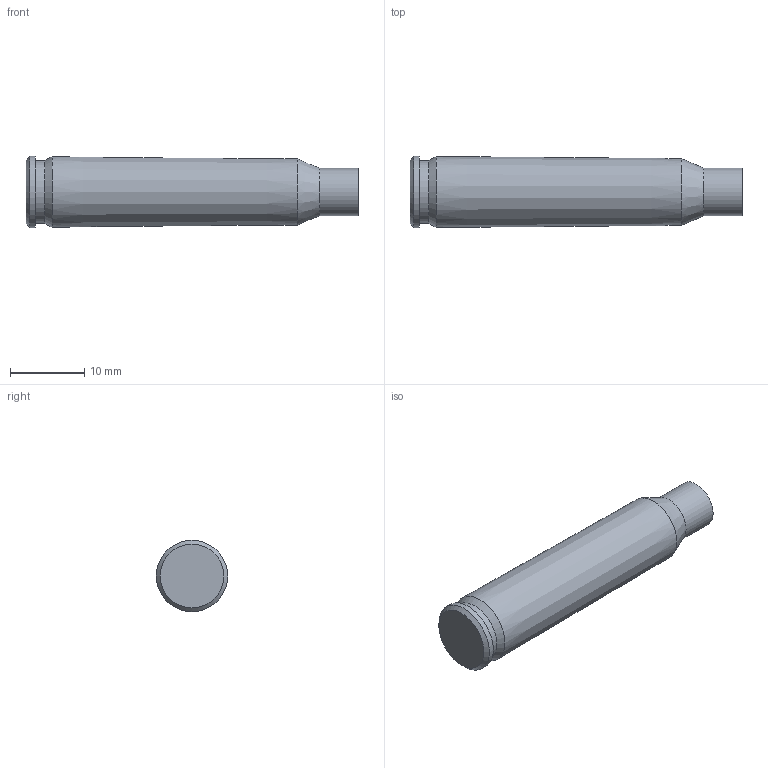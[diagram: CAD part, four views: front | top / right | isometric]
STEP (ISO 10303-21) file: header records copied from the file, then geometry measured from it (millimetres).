
FILE_DESCRIPTION( ( '' ), ' ' );
FILE_NAME( '5a114c57a0eac20dd83200d1.step', '2017-11-19T09:18:16', ( '' ), ( '' ), ' ', ' ', ' ' );
FILE_SCHEMA( ( 'AUTOMOTIVE_DESIGN { 1 0 10303 214 1 1 1 1 }' ) );
Length unit declared in the file: metre
Products named in the file (1): Part 1
Bounding box: 44.7 x 9.6 x 9.6 mm (x, y, z)
Volume: 389.2 mm3; surface area: 2559.6 mm2
Topology: 1 solids, 1 shells, 19 faces, 35 edges, 21 vertices
Faces by surface type: cone 8, cylinder 6, plane 5
Full cylindrical faces by diameter (mm): 5.817 x1, 6.426 x1, 7.823 x1, 8.433 x1, 8.992 x1, 9.601 x1
Entity records: 542 total; most frequent: DIRECTION 76, CARTESIAN_POINT 56, AXIS2_PLACEMENT_3D 38, EDGE_LOOP 36, ORIENTED_EDGE 36, FACE_OUTER_BOUND 25, STYLED_ITEM 19, PRESENTATION_STYLE_ASSIGNMENT 19
